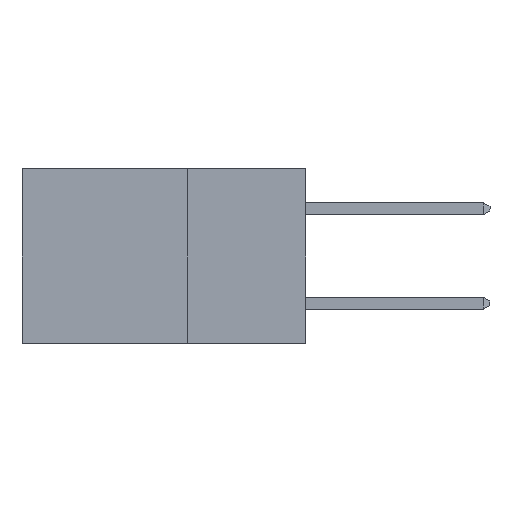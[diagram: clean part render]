
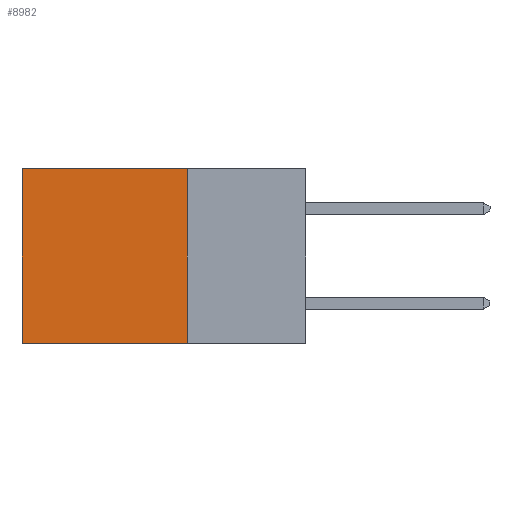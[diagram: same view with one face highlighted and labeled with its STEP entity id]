
A CAD part, left-side view. The second image highlights one B-rep face of the part: STEP entity #8982.
In plain terms, the highlighted planar face has unit normal (-1, 0, 0).
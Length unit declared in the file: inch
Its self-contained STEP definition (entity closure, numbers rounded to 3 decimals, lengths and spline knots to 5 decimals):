
#207 = EDGE_LOOP ( 'NONE', ( #3249, #3151, #3829, #7860 ) ) ;
#380 = PLANE ( 'NONE',  #3712 ) ;
#550 = VECTOR ( 'NONE', #8601, 39.37008 ) ;
#1007 = EDGE_CURVE ( 'NONE', #7742, #8096, #1931, .T. ) ;
#1114 = VECTOR ( 'NONE', #1963, 39.37008 ) ;
#1206 = CARTESIAN_POINT ( 'NONE',  ( 0.2615, 0.25, 0. ) ) ;
#1241 = DIRECTION ( 'NONE',  ( 0., 1., 0. ) ) ;
#1931 = LINE ( 'NONE', #8261, #5299 ) ;
#1963 = DIRECTION ( 'NONE',  ( 0., 1., 0. ) ) ;
#2222 = LINE ( 'NONE', #4845, #1114 ) ;
#3095 = LINE ( 'NONE', #3628, #550 ) ;
#3151 = ORIENTED_EDGE ( 'NONE', *, *, #3298, .F. ) ;
#3178 = CARTESIAN_POINT ( 'NONE',  ( 0.2615, 0.25, -0.37 ) ) ;
#3249 = ORIENTED_EDGE ( 'NONE', *, *, #4144, .T. ) ;
#3298 = EDGE_CURVE ( 'NONE', #6832, #3925, #2222, .T. ) ;
#3628 = CARTESIAN_POINT ( 'NONE',  ( 0.2615, 0.25, -0.37 ) ) ;
#3712 = AXIS2_PLACEMENT_3D ( 'NONE', #3178, #8779, #8135 ) ;
#3827 = CARTESIAN_POINT ( 'NONE',  ( 0.2615, 0.6, -0.37 ) ) ;
#3829 = ORIENTED_EDGE ( 'NONE', *, *, #7195, .F. ) ;
#3925 = VERTEX_POINT ( 'NONE', #3827 ) ;
#4144 = EDGE_CURVE ( 'NONE', #8096, #3925, #6983, .T. ) ;
#4845 = CARTESIAN_POINT ( 'NONE',  ( 0.2615, 0.25, -0.37 ) ) ;
#5100 = DIRECTION ( 'NONE',  ( 0., 0., -1. ) ) ;
#5299 = VECTOR ( 'NONE', #1241, 39.37008 ) ;
#6572 = CARTESIAN_POINT ( 'NONE',  ( 0.2615, 0.6, 0. ) ) ;
#6671 = FACE_OUTER_BOUND ( 'NONE', #207, .T. ) ;
#6832 = VERTEX_POINT ( 'NONE', #7545 ) ;
#6983 = LINE ( 'NONE', #7904, #8430 ) ;
#7195 = EDGE_CURVE ( 'NONE', #7742, #6832, #3095, .T. ) ;
#7545 = CARTESIAN_POINT ( 'NONE',  ( 0.2615, 0.25, -0.37 ) ) ;
#7742 = VERTEX_POINT ( 'NONE', #1206 ) ;
#7860 = ORIENTED_EDGE ( 'NONE', *, *, #1007, .T. ) ;
#7904 = CARTESIAN_POINT ( 'NONE',  ( 0.2615, 0.6, -0.37 ) ) ;
#8096 = VERTEX_POINT ( 'NONE', #6572 ) ;
#8135 = DIRECTION ( 'NONE',  ( 0., 0., -1. ) ) ;
#8261 = CARTESIAN_POINT ( 'NONE',  ( 0.2615, 0.25, 0. ) ) ;
#8430 = VECTOR ( 'NONE', #5100, 39.37008 ) ;
#8601 = DIRECTION ( 'NONE',  ( 0., 0., -1. ) ) ;
#8779 = DIRECTION ( 'NONE',  ( 1., 0., 0. ) ) ;
#8982 = ADVANCED_FACE ( 'NONE', ( #6671 ), #380, .F. ) ;
